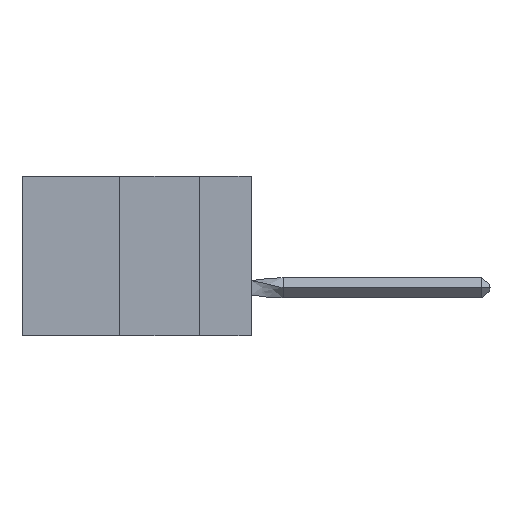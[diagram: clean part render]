
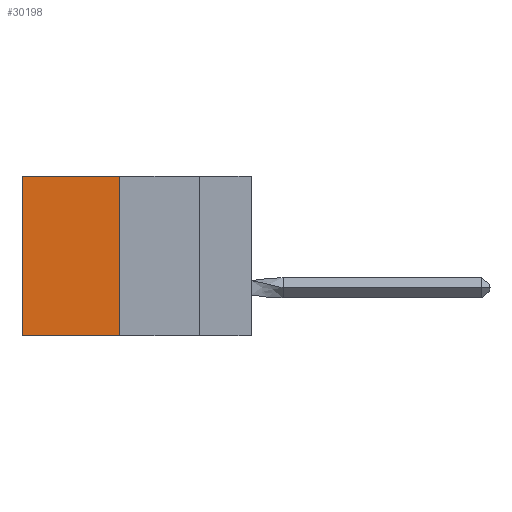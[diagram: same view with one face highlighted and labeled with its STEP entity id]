
A CAD part, left-side view. The second image highlights one B-rep face of the part: STEP entity #30198.
In plain terms, the highlighted planar face has unit normal (-1, 0, 0).
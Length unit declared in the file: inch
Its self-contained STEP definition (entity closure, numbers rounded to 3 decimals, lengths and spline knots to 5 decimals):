
#113 = CARTESIAN_POINT ( 'NONE',  ( 0.305, 0.413, -0.5 ) ) ;
#1957 = VERTEX_POINT ( 'NONE', #113 ) ;
#3260 = EDGE_CURVE ( 'NONE', #22049, #11977, #27695, .T. ) ;
#3465 = FACE_OUTER_BOUND ( 'NONE', #5669, .T. ) ;
#3633 = PLANE ( 'NONE',  #27808 ) ;
#3647 = CARTESIAN_POINT ( 'NONE',  ( 0.305, 0.72, 0. ) ) ;
#5669 = EDGE_LOOP ( 'NONE', ( #16460, #30938, #31664, #21513 ) ) ;
#5867 = DIRECTION ( 'NONE',  ( 1., 0., 0. ) ) ;
#8703 = CARTESIAN_POINT ( 'NONE',  ( 0.305, 0.72, -0.5 ) ) ;
#9611 = EDGE_CURVE ( 'NONE', #1957, #33278, #19239, .T. ) ;
#11977 = VERTEX_POINT ( 'NONE', #3647 ) ;
#12098 = CARTESIAN_POINT ( 'NONE',  ( 0.305, 0.72, -0.5 ) ) ;
#13100 = VECTOR ( 'NONE', #24083, 39.37008 ) ;
#13482 = EDGE_CURVE ( 'NONE', #11977, #33278, #29937, .T. ) ;
#16071 = DIRECTION ( 'NONE',  ( 0., 1., 0. ) ) ;
#16460 = ORIENTED_EDGE ( 'NONE', *, *, #13482, .T. ) ;
#16663 = CARTESIAN_POINT ( 'NONE',  ( 0.305, 0.413, -0.5 ) ) ;
#17187 = EDGE_CURVE ( 'NONE', #22049, #1957, #21096, .T. ) ;
#19239 = LINE ( 'NONE', #31897, #13100 ) ;
#20734 = VECTOR ( 'NONE', #16071, 39.37008 ) ;
#21096 = LINE ( 'NONE', #30388, #31728 ) ;
#21313 = VECTOR ( 'NONE', #30415, 39.37008 ) ;
#21513 = ORIENTED_EDGE ( 'NONE', *, *, #3260, .T. ) ;
#22049 = VERTEX_POINT ( 'NONE', #32720 ) ;
#24083 = DIRECTION ( 'NONE',  ( 0., 1., 0. ) ) ;
#25220 = DIRECTION ( 'NONE',  ( 0., 0., -1. ) ) ;
#26454 = CARTESIAN_POINT ( 'NONE',  ( 0.305, 0.413, 0. ) ) ;
#27695 = LINE ( 'NONE', #26454, #20734 ) ;
#27808 = AXIS2_PLACEMENT_3D ( 'NONE', #16663, #5867, #29690 ) ;
#29690 = DIRECTION ( 'NONE',  ( 0., 0., -1. ) ) ;
#29937 = LINE ( 'NONE', #12098, #21313 ) ;
#30198 = ADVANCED_FACE ( 'NONE', ( #3465 ), #3633, .F. ) ;
#30388 = CARTESIAN_POINT ( 'NONE',  ( 0.305, 0.413, -0.5 ) ) ;
#30415 = DIRECTION ( 'NONE',  ( 0., 0., -1. ) ) ;
#30938 = ORIENTED_EDGE ( 'NONE', *, *, #9611, .F. ) ;
#31664 = ORIENTED_EDGE ( 'NONE', *, *, #17187, .F. ) ;
#31728 = VECTOR ( 'NONE', #25220, 39.37008 ) ;
#31897 = CARTESIAN_POINT ( 'NONE',  ( 0.305, 0.413, -0.5 ) ) ;
#32720 = CARTESIAN_POINT ( 'NONE',  ( 0.305, 0.413, 0. ) ) ;
#33278 = VERTEX_POINT ( 'NONE', #8703 ) ;
